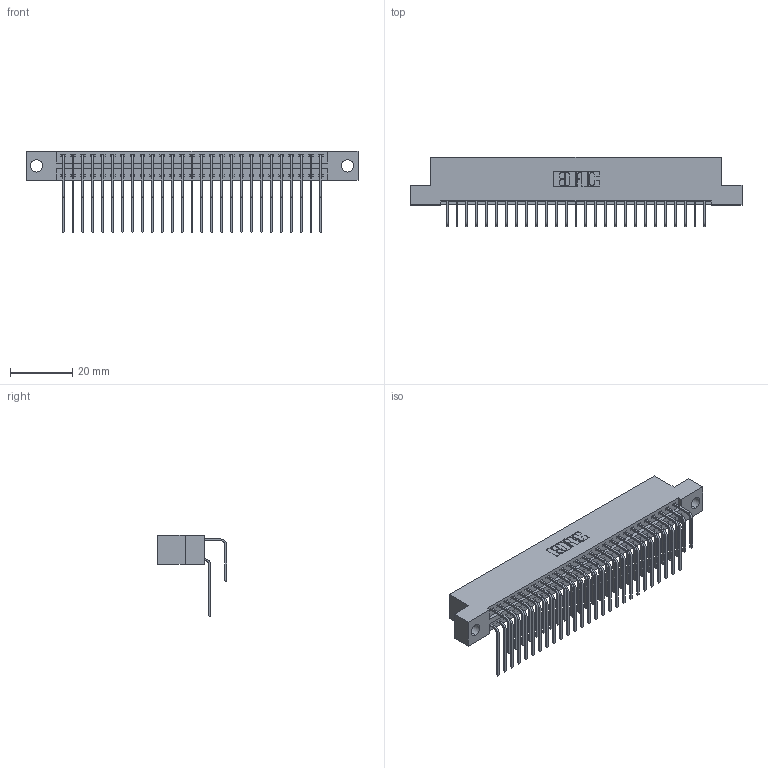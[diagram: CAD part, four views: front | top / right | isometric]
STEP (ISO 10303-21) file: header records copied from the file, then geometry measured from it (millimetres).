
FILE_DESCRIPTION (( 'STEP AP203' ), '1' );
FILE_NAME ('396-054-558-204.STEP', '2018-09-08T08:35:39', ( '' ), ( '' ), 'SwSTEP 2.0', 'SolidWorks 2016', '' );
FILE_SCHEMA (( 'CONFIG_CONTROL_DESIGN' ));
Length unit declared in the file: inch
Products named in the file (4): 346 Part_Flush Mounting Lugs - 0.156 Dia-TH; 345-292-001_558 559 Tail - 1; 345-292-001_558 Tail - 2; 396-054-558-204
Assembly tree (55 placements, depth 2):
  396-054-558-204
    346 Part_Flush Mounting Lugs - 0.156 Dia-TH
    345-292-001_558 559 Tail - 1  x27
    345-292-001_558 Tail - 2  x27
Bounding box: 106.3 x 22.16 x 26.16 mm (x, y, z)
Volume: 10472.6 mm3; surface area: 15467.3 mm2
Topology: 55 solids, 55 shells, 3038 faces, 9023 edges, 5942 vertices
Faces by surface type: plane 2074, cylinder 964
Entity records: 21427 total; most frequent: CARTESIAN_POINT 3603, ORIENTED_EDGE 3486, DIRECTION 3199, EDGE_CURVE 1743, LINE 1463, VECTOR 1463, VERTEX_POINT 1158, AXIS2_PLACEMENT_3D 868
